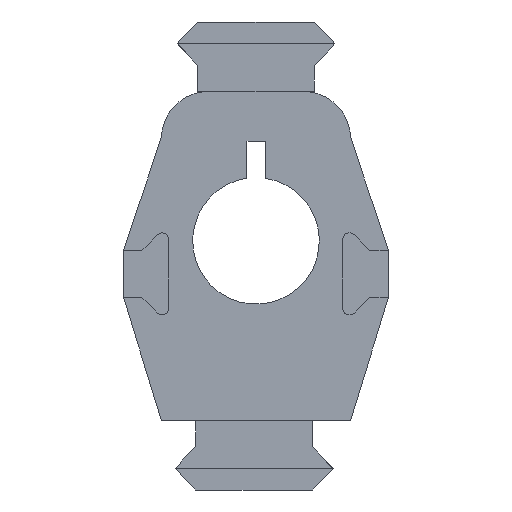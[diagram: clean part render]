
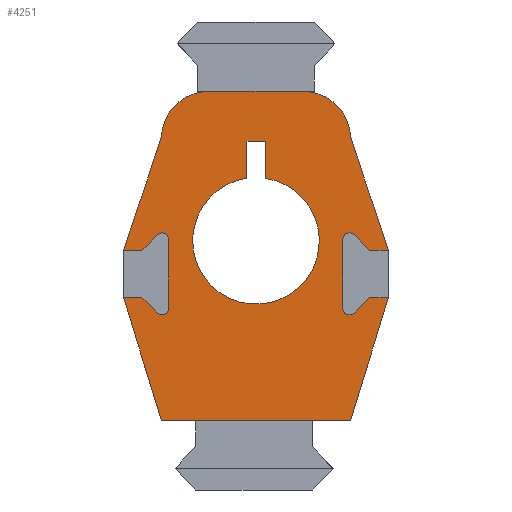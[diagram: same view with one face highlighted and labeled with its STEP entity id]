
A CAD part, front view. The second image highlights one B-rep face of the part: STEP entity #4251.
In plain terms, the highlighted planar face has unit normal (0, -1, 0).
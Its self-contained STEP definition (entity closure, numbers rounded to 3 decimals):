
#14=FACE_BOUND('',#494,.T.);
#37=CIRCLE('',#4497,8.5);
#38=CIRCLE('',#4500,6.35);
#39=CIRCLE('',#4503,6.35);
#40=CIRCLE('',#4510,0.889);
#41=CIRCLE('',#4511,0.889);
#42=CIRCLE('',#4512,0.889);
#43=CIRCLE('',#4513,0.889);
#266=FACE_OUTER_BOUND('',#493,.T.);
#493=EDGE_LOOP('',(#3722,#3723,#3724,#3725,#3726,#3727,#3728,#3729,#3730,
#3731,#3732,#3733,#3734,#3735,#3736,#3737,#3738,#3739,#3740,#3741,#3742,
#3743,#3744,#3745));
#494=EDGE_LOOP('',(#3746,#3747,#3748,#3749));
#1017=LINE('',#6646,#1591);
#1030=LINE('',#6678,#1604);
#1033=LINE('',#6683,#1607);
#1035=LINE('',#6687,#1609);
#1037=LINE('',#6693,#1611);
#1040=LINE('',#6701,#1614);
#1042=LINE('',#6708,#1616);
#1045=LINE('',#6713,#1619);
#1047=LINE('',#6717,#1621);
#1049=LINE('',#6721,#1623);
#1051=LINE('',#6724,#1625);
#1052=LINE('',#6727,#1626);
#1053=LINE('',#6729,#1627);
#1054=LINE('',#6733,#1628);
#1055=LINE('',#6737,#1629);
#1056=LINE('',#6738,#1630);
#1057=LINE('',#6740,#1631);
#1058=LINE('',#6742,#1632);
#1059=LINE('',#6746,#1633);
#1060=LINE('',#6750,#1634);
#1061=LINE('',#6751,#1635);
#1591=VECTOR('',#5446,10.);
#1604=VECTOR('',#5469,10.);
#1607=VECTOR('',#5474,10.);
#1609=VECTOR('',#5478,10.);
#1611=VECTOR('',#5486,10.);
#1614=VECTOR('',#5495,10.);
#1616=VECTOR('',#5503,10.);
#1619=VECTOR('',#5508,10.);
#1621=VECTOR('',#5512,10.);
#1623=VECTOR('',#5516,10.);
#1625=VECTOR('',#5520,10.);
#1626=VECTOR('',#5523,10.);
#1627=VECTOR('',#5524,10.);
#1628=VECTOR('',#5527,10.);
#1629=VECTOR('',#5530,10.);
#1630=VECTOR('',#5531,10.);
#1631=VECTOR('',#5532,10.);
#1632=VECTOR('',#5533,10.);
#1633=VECTOR('',#5536,10.);
#1634=VECTOR('',#5539,10.);
#1635=VECTOR('',#5540,10.);
#1983=VERTEX_POINT('',#6629);
#1986=VERTEX_POINT('',#6635);
#1989=VERTEX_POINT('',#6643);
#1990=VERTEX_POINT('',#6645);
#2003=VERTEX_POINT('',#6676);
#2004=VERTEX_POINT('',#6677);
#2005=VERTEX_POINT('',#6682);
#2006=VERTEX_POINT('',#6686);
#2007=VERTEX_POINT('',#6692);
#2008=VERTEX_POINT('',#6696);
#2009=VERTEX_POINT('',#6700);
#2010=VERTEX_POINT('',#6706);
#2011=VERTEX_POINT('',#6707);
#2012=VERTEX_POINT('',#6712);
#2013=VERTEX_POINT('',#6716);
#2014=VERTEX_POINT('',#6720);
#2015=VERTEX_POINT('',#6726);
#2016=VERTEX_POINT('',#6728);
#2017=VERTEX_POINT('',#6730);
#2018=VERTEX_POINT('',#6732);
#2019=VERTEX_POINT('',#6734);
#2020=VERTEX_POINT('',#6736);
#2021=VERTEX_POINT('',#6739);
#2022=VERTEX_POINT('',#6741);
#2023=VERTEX_POINT('',#6743);
#2024=VERTEX_POINT('',#6745);
#2025=VERTEX_POINT('',#6747);
#2026=VERTEX_POINT('',#6749);
#2553=EDGE_CURVE('',#1989,#1990,#1017,.T.);
#2569=EDGE_CURVE('',#2003,#2004,#1030,.T.);
#2572=EDGE_CURVE('',#2005,#2003,#1033,.T.);
#2574=EDGE_CURVE('',#2006,#2005,#1035,.T.);
#2576=EDGE_CURVE('',#2004,#2006,#37,.T.);
#2577=EDGE_CURVE('',#2007,#1983,#1037,.T.);
#2579=EDGE_CURVE('',#2008,#2007,#38,.T.);
#2581=EDGE_CURVE('',#2009,#2008,#1040,.T.);
#2583=EDGE_CURVE('',#1990,#2009,#39,.T.);
#2584=EDGE_CURVE('',#2010,#2011,#1042,.T.);
#2587=EDGE_CURVE('',#2012,#2010,#1045,.T.);
#2589=EDGE_CURVE('',#2013,#2012,#1047,.T.);
#2591=EDGE_CURVE('',#2014,#2013,#1049,.T.);
#2593=EDGE_CURVE('',#1986,#2014,#1051,.T.);
#2594=EDGE_CURVE('',#2015,#1986,#1052,.T.);
#2595=EDGE_CURVE('',#2016,#2015,#1053,.T.);
#2596=EDGE_CURVE('',#2017,#2016,#40,.T.);
#2597=EDGE_CURVE('',#2018,#2017,#1054,.T.);
#2598=EDGE_CURVE('',#2019,#2018,#41,.T.);
#2599=EDGE_CURVE('',#2020,#2019,#1055,.T.);
#2600=EDGE_CURVE('',#1983,#2020,#1056,.T.);
#2601=EDGE_CURVE('',#2021,#1989,#1057,.T.);
#2602=EDGE_CURVE('',#2022,#2021,#1058,.T.);
#2603=EDGE_CURVE('',#2023,#2022,#42,.T.);
#2604=EDGE_CURVE('',#2024,#2023,#1059,.T.);
#2605=EDGE_CURVE('',#2025,#2024,#43,.T.);
#2606=EDGE_CURVE('',#2026,#2025,#1060,.T.);
#2607=EDGE_CURVE('',#2011,#2026,#1061,.T.);
#3722=ORIENTED_EDGE('',*,*,#2593,.F.);
#3723=ORIENTED_EDGE('',*,*,#2594,.F.);
#3724=ORIENTED_EDGE('',*,*,#2595,.F.);
#3725=ORIENTED_EDGE('',*,*,#2596,.F.);
#3726=ORIENTED_EDGE('',*,*,#2597,.F.);
#3727=ORIENTED_EDGE('',*,*,#2598,.F.);
#3728=ORIENTED_EDGE('',*,*,#2599,.F.);
#3729=ORIENTED_EDGE('',*,*,#2600,.F.);
#3730=ORIENTED_EDGE('',*,*,#2577,.F.);
#3731=ORIENTED_EDGE('',*,*,#2579,.F.);
#3732=ORIENTED_EDGE('',*,*,#2581,.F.);
#3733=ORIENTED_EDGE('',*,*,#2583,.F.);
#3734=ORIENTED_EDGE('',*,*,#2553,.F.);
#3735=ORIENTED_EDGE('',*,*,#2601,.F.);
#3736=ORIENTED_EDGE('',*,*,#2602,.F.);
#3737=ORIENTED_EDGE('',*,*,#2603,.F.);
#3738=ORIENTED_EDGE('',*,*,#2604,.F.);
#3739=ORIENTED_EDGE('',*,*,#2605,.F.);
#3740=ORIENTED_EDGE('',*,*,#2606,.F.);
#3741=ORIENTED_EDGE('',*,*,#2607,.F.);
#3742=ORIENTED_EDGE('',*,*,#2584,.F.);
#3743=ORIENTED_EDGE('',*,*,#2587,.F.);
#3744=ORIENTED_EDGE('',*,*,#2589,.F.);
#3745=ORIENTED_EDGE('',*,*,#2591,.F.);
#3746=ORIENTED_EDGE('',*,*,#2576,.F.);
#3747=ORIENTED_EDGE('',*,*,#2569,.F.);
#3748=ORIENTED_EDGE('',*,*,#2572,.F.);
#3749=ORIENTED_EDGE('',*,*,#2574,.F.);
#4029=PLANE('',#4509);
#4251=ADVANCED_FACE('',(#266,#14),#4029,.F.);
#4497=AXIS2_PLACEMENT_3D('',#6690,#5482,#5483);
#4500=AXIS2_PLACEMENT_3D('',#6697,#5490,#5491);
#4503=AXIS2_PLACEMENT_3D('',#6704,#5499,#5500);
#4509=AXIS2_PLACEMENT_3D('',#6725,#5521,#5522);
#4510=AXIS2_PLACEMENT_3D('',#6731,#5525,#5526);
#4511=AXIS2_PLACEMENT_3D('',#6735,#5528,#5529);
#4512=AXIS2_PLACEMENT_3D('',#6744,#5534,#5535);
#4513=AXIS2_PLACEMENT_3D('',#6748,#5537,#5538);
#5446=DIRECTION('',(0.316,0.,0.949));
#5469=DIRECTION('',(0.,0.,-1.));
#5474=DIRECTION('',(-1.,0.,0.));
#5478=DIRECTION('',(0.,0.,1.));
#5482=DIRECTION('center_axis',(0.,-1.,0.));
#5483=DIRECTION('ref_axis',(-1.,0.,0.));
#5486=DIRECTION('',(0.316,0.,-0.949));
#5490=DIRECTION('center_axis',(0.,1.,0.));
#5491=DIRECTION('ref_axis',(0.999,0.,0.04));
#5495=DIRECTION('',(1.,0.,0.));
#5499=DIRECTION('center_axis',(0.,1.,0.));
#5500=DIRECTION('ref_axis',(-0.999,0.,0.04));
#5503=DIRECTION('',(-0.294,0.,0.956));
#5508=DIRECTION('',(0.,0.,-1.));
#5512=DIRECTION('',(-1.,0.,0.));
#5516=DIRECTION('',(0.,0.,1.));
#5520=DIRECTION('',(-0.294,0.,-0.956));
#5521=DIRECTION('center_axis',(0.,1.,0.));
#5522=DIRECTION('ref_axis',(-1.,0.,0.));
#5523=DIRECTION('',(1.,0.,0.));
#5524=DIRECTION('',(0.707,0.,0.707));
#5525=DIRECTION('center_axis',(0.,-1.,0.));
#5526=DIRECTION('ref_axis',(0.707,0.,-0.707));
#5527=DIRECTION('',(0.,0.,-1.));
#5528=DIRECTION('center_axis',(0.,-1.,0.));
#5529=DIRECTION('ref_axis',(-1.,0.,0.));
#5530=DIRECTION('',(-0.707,0.,0.707));
#5531=DIRECTION('',(-1.,0.,0.001));
#5532=DIRECTION('',(-1.,0.,-0.001));
#5533=DIRECTION('',(-0.707,0.,-0.707));
#5534=DIRECTION('center_axis',(0.,-1.,0.));
#5535=DIRECTION('ref_axis',(-0.707,0.,0.707));
#5536=DIRECTION('',(0.,0.,1.));
#5537=DIRECTION('center_axis',(0.,-1.,0.));
#5538=DIRECTION('ref_axis',(1.,0.,0.));
#5539=DIRECTION('',(0.707,0.,-0.707));
#5540=DIRECTION('',(1.,0.,0.));
#6629=CARTESIAN_POINT('',(17.78,348.84,10.16));
#6635=CARTESIAN_POINT('',(17.78,348.84,3.81));
#6643=CARTESIAN_POINT('',(-17.78,348.84,10.16));
#6645=CARTESIAN_POINT('',(-12.7,348.84,25.4));
#6646=CARTESIAN_POINT('',(-18.105,348.84,9.186));
#6676=CARTESIAN_POINT('',(-1.212,348.84,24.821));
#6677=CARTESIAN_POINT('',(-1.212,348.84,19.843));
#6678=CARTESIAN_POINT('',(-1.212,348.84,13.085));
#6682=CARTESIAN_POINT('',(1.288,348.84,24.821));
#6683=CARTESIAN_POINT('',(0.644,348.84,24.821));
#6686=CARTESIAN_POINT('',(1.288,348.84,19.832));
#6687=CARTESIAN_POINT('',(1.288,348.84,13.085));
#6690=CARTESIAN_POINT('Origin',(0.,348.84,11.43));
#6692=CARTESIAN_POINT('',(12.7,348.84,25.4));
#6693=CARTESIAN_POINT('',(14.923,348.84,18.733));
#6696=CARTESIAN_POINT('',(6.355,348.84,31.496));
#6697=CARTESIAN_POINT('Origin',(6.355,348.84,25.146));
#6700=CARTESIAN_POINT('',(-6.355,348.84,31.496));
#6701=CARTESIAN_POINT('',(-6.35,348.84,31.496));
#6704=CARTESIAN_POINT('Origin',(-6.355,348.84,25.146));
#6706=CARTESIAN_POINT('',(-12.7,348.84,-12.7));
#6707=CARTESIAN_POINT('',(-17.78,348.84,3.81));
#6708=CARTESIAN_POINT('',(-14.828,348.84,-5.784));
#6712=CARTESIAN_POINT('',(-12.7,348.84,-12.699));
#6713=CARTESIAN_POINT('',(-12.7,348.84,-3.175));
#6716=CARTESIAN_POINT('',(12.7,348.84,-12.699));
#6717=CARTESIAN_POINT('',(-6.35,348.84,-12.699));
#6720=CARTESIAN_POINT('',(12.7,348.84,-12.7));
#6721=CARTESIAN_POINT('',(12.7,348.84,-3.175));
#6724=CARTESIAN_POINT('',(17.368,348.84,2.471));
#6725=CARTESIAN_POINT('Origin',(-14.753,348.84,6.987));
#6726=CARTESIAN_POINT('',(15.24,348.84,3.81));
#6727=CARTESIAN_POINT('',(1.514,348.84,3.81));
#6728=CARTESIAN_POINT('',(13.166,348.84,1.736));
#6729=CARTESIAN_POINT('',(8.536,348.84,-2.894));
#6730=CARTESIAN_POINT('',(11.648,348.84,2.364));
#6731=CARTESIAN_POINT('Origin',(12.537,348.84,2.364));
#6732=CARTESIAN_POINT('',(11.648,348.84,11.609));
#6733=CARTESIAN_POINT('',(11.648,348.84,4.675));
#6734=CARTESIAN_POINT('',(13.166,348.84,12.238));
#6735=CARTESIAN_POINT('Origin',(12.537,348.84,11.609));
#6736=CARTESIAN_POINT('',(15.24,348.84,10.163));
#6737=CARTESIAN_POINT('',(7.499,348.84,17.904));
#6738=CARTESIAN_POINT('',(0.246,348.84,10.181));
#6739=CARTESIAN_POINT('',(-15.317,348.84,10.163));
#6740=CARTESIAN_POINT('',(-16.268,348.84,10.162));
#6741=CARTESIAN_POINT('',(-13.243,348.84,12.238));
#6742=CARTESIAN_POINT('',(-15.97,348.84,9.51));
#6743=CARTESIAN_POINT('',(-11.725,348.84,11.609));
#6744=CARTESIAN_POINT('Origin',(-12.614,348.84,11.609));
#6745=CARTESIAN_POINT('',(-11.725,348.84,2.364));
#6746=CARTESIAN_POINT('',(-11.725,348.84,9.298));
#6747=CARTESIAN_POINT('',(-13.243,348.84,1.736));
#6748=CARTESIAN_POINT('Origin',(-12.614,348.84,2.364));
#6749=CARTESIAN_POINT('',(-15.317,348.84,3.81));
#6750=CARTESIAN_POINT('',(-14.933,348.84,3.426));
#6751=CARTESIAN_POINT('',(-15.035,348.84,3.81));
